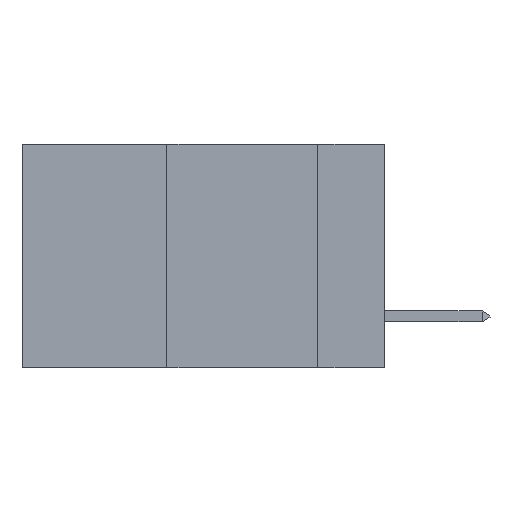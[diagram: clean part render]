
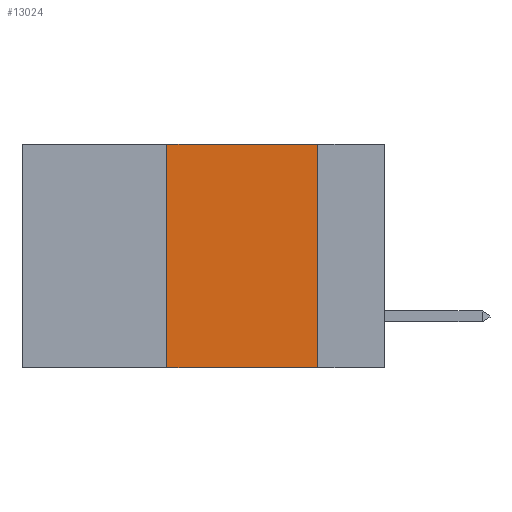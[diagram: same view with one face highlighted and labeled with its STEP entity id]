
A CAD part, left-side view. The second image highlights one B-rep face of the part: STEP entity #13024.
In plain terms, the highlighted planar face has unit normal (-1, 0, 0).
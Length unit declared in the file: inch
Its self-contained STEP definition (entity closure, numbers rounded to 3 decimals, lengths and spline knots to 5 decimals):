
#112 = AXIS2_PLACEMENT_3D ( 'NONE', #6957, #20379, #8898 ) ;
#155 = EDGE_CURVE ( 'NONE', #17746, #9769, #21423, .T. ) ;
#2974 = PLANE ( 'NONE',  #112 ) ;
#3420 = EDGE_LOOP ( 'NONE', ( #15413, #16460, #14977, #23064 ) ) ;
#4008 = CARTESIAN_POINT ( 'NONE',  ( 0., 0.36, -0.37 ) ) ;
#4964 = VECTOR ( 'NONE', #10851, 39.37008 ) ;
#6055 = VECTOR ( 'NONE', #13659, 39.37008 ) ;
#6099 = VECTOR ( 'NONE', #8835, 39.37008 ) ;
#6271 = VERTEX_POINT ( 'NONE', #15717 ) ;
#6957 = CARTESIAN_POINT ( 'NONE',  ( 0., 0.6, 0. ) ) ;
#7234 = CARTESIAN_POINT ( 'NONE',  ( 0., 0.36, 0. ) ) ;
#7517 = CARTESIAN_POINT ( 'NONE',  ( 0., 0.36, 0. ) ) ;
#8567 = DIRECTION ( 'NONE',  ( 0., -1., 0. ) ) ;
#8762 = CARTESIAN_POINT ( 'NONE',  ( 0., 0.11, 0. ) ) ;
#8835 = DIRECTION ( 'NONE',  ( 0., 0., 1. ) ) ;
#8898 = DIRECTION ( 'NONE',  ( 0., 0., -1. ) ) ;
#9210 = CARTESIAN_POINT ( 'NONE',  ( 0., 0.11, 0. ) ) ;
#9769 = VERTEX_POINT ( 'NONE', #7517 ) ;
#10154 = LINE ( 'NONE', #8762, #4964 ) ;
#10463 = CARTESIAN_POINT ( 'NONE',  ( 0., 0.6, 0. ) ) ;
#10851 = DIRECTION ( 'NONE',  ( 0., 0., -1. ) ) ;
#11733 = CARTESIAN_POINT ( 'NONE',  ( 0., 0.6, -0.37 ) ) ;
#12125 = EDGE_CURVE ( 'NONE', #23327, #6271, #10154, .T. ) ;
#12916 = EDGE_CURVE ( 'NONE', #9769, #23327, #21464, .T. ) ;
#13024 = ADVANCED_FACE ( 'NONE', ( #23550 ), #2974, .F. ) ;
#13659 = DIRECTION ( 'NONE',  ( 0., -1., 0. ) ) ;
#14977 = ORIENTED_EDGE ( 'NONE', *, *, #155, .F. ) ;
#15413 = ORIENTED_EDGE ( 'NONE', *, *, #12125, .F. ) ;
#15717 = CARTESIAN_POINT ( 'NONE',  ( 0., 0.11, -0.37 ) ) ;
#16373 = LINE ( 'NONE', #11733, #6055 ) ;
#16460 = ORIENTED_EDGE ( 'NONE', *, *, #12916, .F. ) ;
#17746 = VERTEX_POINT ( 'NONE', #4008 ) ;
#18155 = EDGE_CURVE ( 'NONE', #17746, #6271, #16373, .T. ) ;
#20379 = DIRECTION ( 'NONE',  ( 1., 0., 0. ) ) ;
#20864 = VECTOR ( 'NONE', #8567, 39.37008 ) ;
#21423 = LINE ( 'NONE', #7234, #6099 ) ;
#21464 = LINE ( 'NONE', #10463, #20864 ) ;
#23064 = ORIENTED_EDGE ( 'NONE', *, *, #18155, .T. ) ;
#23327 = VERTEX_POINT ( 'NONE', #9210 ) ;
#23550 = FACE_OUTER_BOUND ( 'NONE', #3420, .T. ) ;
